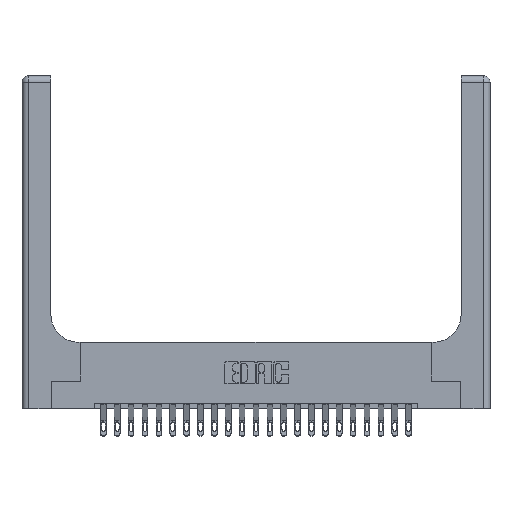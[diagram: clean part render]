
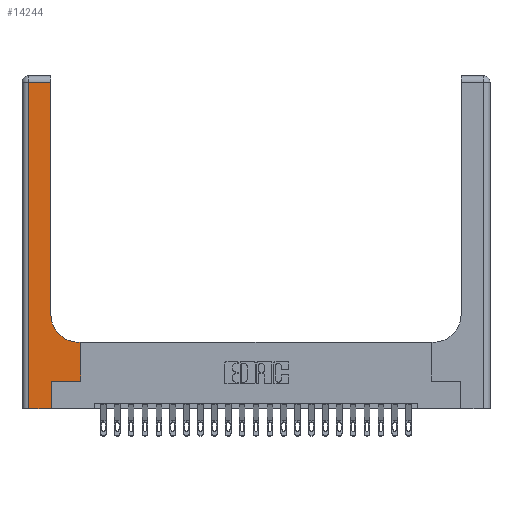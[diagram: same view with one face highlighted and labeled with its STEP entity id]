
A CAD part, top view. The second image highlights one B-rep face of the part: STEP entity #14244.
In plain terms, the highlighted planar face has unit normal (0, 0, 1).
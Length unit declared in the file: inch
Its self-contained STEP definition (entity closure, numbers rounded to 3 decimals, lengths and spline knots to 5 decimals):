
#153 = VERTEX_POINT ( 'NONE', #11632 ) ;
#398 = CARTESIAN_POINT ( 'NONE',  ( 0.26, 0.6, 0.37 ) ) ;
#589 = CARTESIAN_POINT ( 'NONE',  ( 0., 0., 0.37 ) ) ;
#743 = LINE ( 'NONE', #5377, #16103 ) ;
#999 = VECTOR ( 'NONE', #2380, 39.37008 ) ;
#1010 = CARTESIAN_POINT ( 'NONE',  ( 0.06, 0., 0.37 ) ) ;
#1611 = LINE ( 'NONE', #398, #21677 ) ;
#1786 = EDGE_LOOP ( 'NONE', ( #17379, #9347, #7049, #12669, #7121, #6809, #15986, #21650, #6658 ) ) ;
#1937 = EDGE_CURVE ( 'NONE', #153, #8466, #4540, .T. ) ;
#2380 = DIRECTION ( 'NONE',  ( 1., 0., 0. ) ) ;
#2419 = LINE ( 'NONE', #20957, #13841 ) ;
#2502 = CARTESIAN_POINT ( 'NONE',  ( 0.528, 0.6, 0.37 ) ) ;
#2935 = EDGE_CURVE ( 'NONE', #15625, #153, #10340, .T. ) ;
#4053 = VECTOR ( 'NONE', #7951, 39.37008 ) ;
#4540 = LINE ( 'NONE', #22192, #21846 ) ;
#5078 = VERTEX_POINT ( 'NONE', #19025 ) ;
#5130 = CARTESIAN_POINT ( 'NONE',  ( 0.265, 0., 0.37 ) ) ;
#5140 = AXIS2_PLACEMENT_3D ( 'NONE', #18515, #7960, #15064 ) ;
#5377 = CARTESIAN_POINT ( 'NONE',  ( 0.265, 0., 0.37 ) ) ;
#5766 = EDGE_CURVE ( 'NONE', #20712, #19936, #743, .T. ) ;
#6065 = CARTESIAN_POINT ( 'NONE',  ( 0.528, 0.25, 0.37 ) ) ;
#6413 = VERTEX_POINT ( 'NONE', #1010 ) ;
#6445 = EDGE_CURVE ( 'NONE', #8466, #6413, #2419, .T. ) ;
#6658 = ORIENTED_EDGE ( 'NONE', *, *, #20997, .T. ) ;
#6713 = CARTESIAN_POINT ( 'NONE',  ( 0.26, 0.85, 0.37 ) ) ;
#6809 = ORIENTED_EDGE ( 'NONE', *, *, #18784, .T. ) ;
#7049 = ORIENTED_EDGE ( 'NONE', *, *, #6445, .T. ) ;
#7076 = EDGE_CURVE ( 'NONE', #5078, #21308, #21902, .T. ) ;
#7121 = ORIENTED_EDGE ( 'NONE', *, *, #5766, .T. ) ;
#7862 = CARTESIAN_POINT ( 'NONE',  ( 0.265, 0.25, 0.37 ) ) ;
#7951 = DIRECTION ( 'NONE',  ( 0., 1., 0. ) ) ;
#7960 = DIRECTION ( 'NONE',  ( 0., 0., -1. ) ) ;
#8093 = DIRECTION ( 'NONE',  ( 1., 0., 0. ) ) ;
#8466 = VERTEX_POINT ( 'NONE', #17565 ) ;
#9255 = DIRECTION ( 'NONE',  ( 0., 1., 0. ) ) ;
#9318 = CARTESIAN_POINT ( 'NONE',  ( 0.51, 0.85, 0.37 ) ) ;
#9347 = ORIENTED_EDGE ( 'NONE', *, *, #1937, .T. ) ;
#9515 = PLANE ( 'NONE',  #5140 ) ;
#9558 = DIRECTION ( 'NONE',  ( 1., 0., 0. ) ) ;
#9672 = FACE_OUTER_BOUND ( 'NONE', #1786, .T. ) ;
#10340 = LINE ( 'NONE', #16309, #11764 ) ;
#10481 = LINE ( 'NONE', #589, #999 ) ;
#11566 = CARTESIAN_POINT ( 'NONE',  ( 0.265, 0.25, 0.37 ) ) ;
#11632 = CARTESIAN_POINT ( 'NONE',  ( 0.26, 2.94, 0.37 ) ) ;
#11764 = VECTOR ( 'NONE', #9255, 39.37008 ) ;
#12206 = CIRCLE ( 'NONE', #17711, 0.25 ) ;
#12578 = LINE ( 'NONE', #7862, #19024 ) ;
#12669 = ORIENTED_EDGE ( 'NONE', *, *, #22579, .T. ) ;
#13841 = VECTOR ( 'NONE', #15664, 39.37008 ) ;
#14244 = ADVANCED_FACE ( 'NONE', ( #9672 ), #9515, .F. ) ;
#14339 = EDGE_CURVE ( 'NONE', #21308, #16237, #1611, .T. ) ;
#15064 = DIRECTION ( 'NONE',  ( -1., 0., 0. ) ) ;
#15625 = VERTEX_POINT ( 'NONE', #6713 ) ;
#15664 = DIRECTION ( 'NONE',  ( 0., -1., 0. ) ) ;
#15986 = ORIENTED_EDGE ( 'NONE', *, *, #7076, .T. ) ;
#16103 = VECTOR ( 'NONE', #16398, 39.37008 ) ;
#16237 = VERTEX_POINT ( 'NONE', #19093 ) ;
#16309 = CARTESIAN_POINT ( 'NONE',  ( 0.26, 3., 0.37 ) ) ;
#16398 = DIRECTION ( 'NONE',  ( 0., 1., 0. ) ) ;
#16904 = DIRECTION ( 'NONE',  ( -1., 0., 0. ) ) ;
#17379 = ORIENTED_EDGE ( 'NONE', *, *, #2935, .T. ) ;
#17565 = CARTESIAN_POINT ( 'NONE',  ( 0.06, 2.94, 0.37 ) ) ;
#17711 = AXIS2_PLACEMENT_3D ( 'NONE', #9318, #20100, #9558 ) ;
#18515 = CARTESIAN_POINT ( 'NONE',  ( 0., 3., 0.37 ) ) ;
#18784 = EDGE_CURVE ( 'NONE', #19936, #5078, #12578, .T. ) ;
#19024 = VECTOR ( 'NONE', #8093, 39.37008 ) ;
#19025 = CARTESIAN_POINT ( 'NONE',  ( 0.528, 0.25, 0.37 ) ) ;
#19093 = CARTESIAN_POINT ( 'NONE',  ( 0.51, 0.6, 0.37 ) ) ;
#19936 = VERTEX_POINT ( 'NONE', #11566 ) ;
#20100 = DIRECTION ( 'NONE',  ( 0., 0., -1. ) ) ;
#20712 = VERTEX_POINT ( 'NONE', #5130 ) ;
#20957 = CARTESIAN_POINT ( 'NONE',  ( 0.06, 3., 0.37 ) ) ;
#20997 = EDGE_CURVE ( 'NONE', #16237, #15625, #12206, .T. ) ;
#21308 = VERTEX_POINT ( 'NONE', #2502 ) ;
#21650 = ORIENTED_EDGE ( 'NONE', *, *, #14339, .T. ) ;
#21677 = VECTOR ( 'NONE', #21816, 39.37008 ) ;
#21816 = DIRECTION ( 'NONE',  ( -1., 0., 0. ) ) ;
#21846 = VECTOR ( 'NONE', #16904, 39.37008 ) ;
#21902 = LINE ( 'NONE', #6065, #4053 ) ;
#22192 = CARTESIAN_POINT ( 'NONE',  ( 0., 2.94, 0.37 ) ) ;
#22579 = EDGE_CURVE ( 'NONE', #6413, #20712, #10481, .T. ) ;
